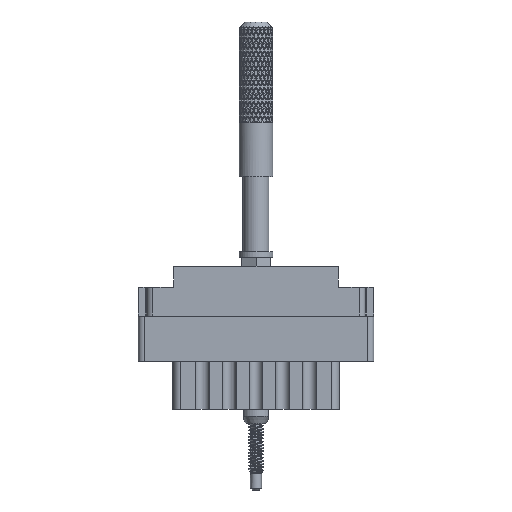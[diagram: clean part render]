
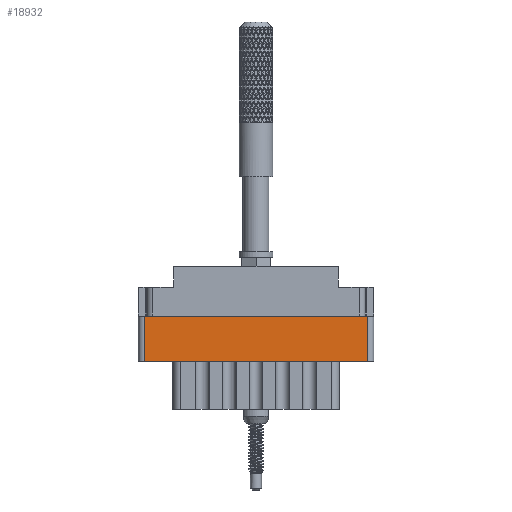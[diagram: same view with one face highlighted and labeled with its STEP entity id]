
A CAD part, front view. The second image highlights one B-rep face of the part: STEP entity #18932.
In plain terms, the highlighted planar face has unit normal (0, -1, 0).
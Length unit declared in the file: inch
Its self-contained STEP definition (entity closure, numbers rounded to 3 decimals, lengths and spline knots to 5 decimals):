
#2300 = EDGE_CURVE ( 'NONE', #91344, #9181, #129260, .T. ) ;
#4144 = VECTOR ( 'NONE', #129916, 39.37008 ) ;
#8410 = CARTESIAN_POINT ( 'NONE',  ( 0.624, -0.343, -0.529 ) ) ;
#9181 = VERTEX_POINT ( 'NONE', #93788 ) ;
#10031 = DIRECTION ( 'NONE',  ( 0., 0., -1. ) ) ;
#11819 = PLANE ( 'NONE',  #106884 ) ;
#12158 = ORIENTED_EDGE ( 'NONE', *, *, #172556, .F. ) ;
#12705 = FACE_OUTER_BOUND ( 'NONE', #95033, .T. ) ;
#13473 = DIRECTION ( 'NONE',  ( 0., 0., 1. ) ) ;
#18932 = ADVANCED_FACE ( 'NONE', ( #12705 ), #11819, .T. ) ;
#31652 = EDGE_CURVE ( 'NONE', #152522, #91344, #135967, .T. ) ;
#50294 = LINE ( 'NONE', #8410, #94166 ) ;
#65370 = ORIENTED_EDGE ( 'NONE', *, *, #31652, .F. ) ;
#67137 = ORIENTED_EDGE ( 'NONE', *, *, #96500, .T. ) ;
#68120 = LINE ( 'NONE', #138164, #170183 ) ;
#80413 = ORIENTED_EDGE ( 'NONE', *, *, #2300, .F. ) ;
#91344 = VERTEX_POINT ( 'NONE', #157798 ) ;
#93788 = CARTESIAN_POINT ( 'NONE',  ( 0.624, -0.343, -0.277 ) ) ;
#94166 = VECTOR ( 'NONE', #160444, 39.37008 ) ;
#95033 = EDGE_LOOP ( 'NONE', ( #65370, #12158, #67137, #80413 ) ) ;
#95054 = CARTESIAN_POINT ( 'NONE',  ( -0.624, -0.343, -0.798 ) ) ;
#96500 = EDGE_CURVE ( 'NONE', #149946, #9181, #68120, .T. ) ;
#106884 = AXIS2_PLACEMENT_3D ( 'NONE', #137387, #147511, #10031 ) ;
#111125 = CARTESIAN_POINT ( 'NONE',  ( 0.624, -0.343, -0.529 ) ) ;
#112948 = CARTESIAN_POINT ( 'NONE',  ( -0.656, -0.343, -0.277 ) ) ;
#114746 = DIRECTION ( 'NONE',  ( 1., 0., 0. ) ) ;
#128976 = VECTOR ( 'NONE', #114746, 39.37008 ) ;
#129260 = LINE ( 'NONE', #112948, #128976 ) ;
#129916 = DIRECTION ( 'NONE',  ( 0., 0., 1. ) ) ;
#135967 = LINE ( 'NONE', #95054, #4144 ) ;
#137387 = CARTESIAN_POINT ( 'NONE',  ( -0.624, -0.343, -0.798 ) ) ;
#138164 = CARTESIAN_POINT ( 'NONE',  ( 0.624, -0.343, -0.798 ) ) ;
#147511 = DIRECTION ( 'NONE',  ( 0., -1., 0. ) ) ;
#147973 = CARTESIAN_POINT ( 'NONE',  ( -0.624, -0.343, -0.529 ) ) ;
#149946 = VERTEX_POINT ( 'NONE', #111125 ) ;
#152522 = VERTEX_POINT ( 'NONE', #147973 ) ;
#157798 = CARTESIAN_POINT ( 'NONE',  ( -0.624, -0.343, -0.277 ) ) ;
#160444 = DIRECTION ( 'NONE',  ( -1., 0., 0. ) ) ;
#170183 = VECTOR ( 'NONE', #13473, 39.37008 ) ;
#172556 = EDGE_CURVE ( 'NONE', #149946, #152522, #50294, .T. ) ;
